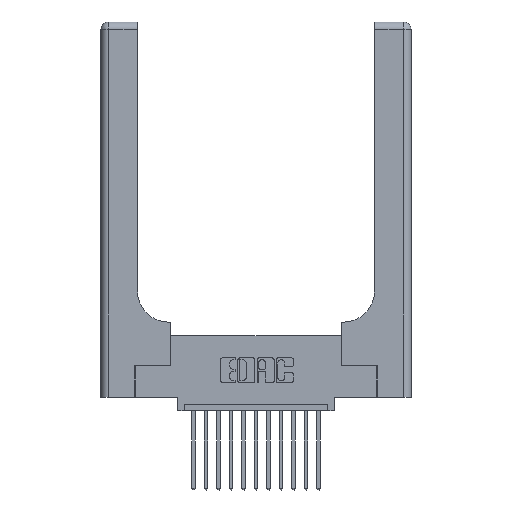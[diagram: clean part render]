
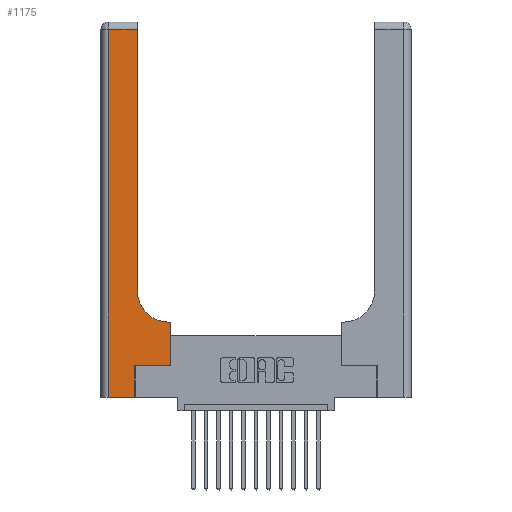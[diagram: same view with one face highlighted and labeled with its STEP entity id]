
A CAD part, top view. The second image highlights one B-rep face of the part: STEP entity #1175.
In plain terms, the highlighted planar face has unit normal (0, 0, 1).
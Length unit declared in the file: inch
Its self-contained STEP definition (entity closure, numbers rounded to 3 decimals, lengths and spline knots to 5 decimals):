
#129 = DIRECTION ( 'NONE',  ( 1., 0., 0. ) ) ;
#448 = PLANE ( 'NONE',  #14762 ) ;
#507 = DIRECTION ( 'NONE',  ( 0., 1., 0. ) ) ;
#669 = VECTOR ( 'NONE', #129, 39.37008 ) ;
#810 = VECTOR ( 'NONE', #507, 39.37008 ) ;
#836 = DIRECTION ( 'NONE',  ( 1., 0., 0. ) ) ;
#1175 = ADVANCED_FACE ( 'NONE', ( #10961 ), #448, .F. ) ;
#1431 = EDGE_CURVE ( 'NONE', #13646, #5494, #13086, .T. ) ;
#1509 = VECTOR ( 'NONE', #16615, 39.37008 ) ;
#1806 = ORIENTED_EDGE ( 'NONE', *, *, #9080, .T. ) ;
#1809 = DIRECTION ( 'NONE',  ( -1., 0., 0. ) ) ;
#2566 = DIRECTION ( 'NONE',  ( 1., 0., 0. ) ) ;
#2981 = VERTEX_POINT ( 'NONE', #3593 ) ;
#3011 = DIRECTION ( 'NONE',  ( 0., 0., -1. ) ) ;
#3562 = DIRECTION ( 'NONE',  ( 0., -1., 0. ) ) ;
#3593 = CARTESIAN_POINT ( 'NONE',  ( 0.06, 0., 0.37 ) ) ;
#3662 = VERTEX_POINT ( 'NONE', #6602 ) ;
#4334 = LINE ( 'NONE', #5508, #669 ) ;
#4370 = ORIENTED_EDGE ( 'NONE', *, *, #8007, .T. ) ;
#4672 = CARTESIAN_POINT ( 'NONE',  ( 0.2915, 3., 0.37 ) ) ;
#4741 = LINE ( 'NONE', #7735, #12445 ) ;
#5181 = EDGE_CURVE ( 'NONE', #10892, #3662, #14459, .T. ) ;
#5494 = VERTEX_POINT ( 'NONE', #14307 ) ;
#5508 = CARTESIAN_POINT ( 'NONE',  ( 0., 0., 0.37 ) ) ;
#5818 = CARTESIAN_POINT ( 'NONE',  ( 0.269, 0., 0.37 ) ) ;
#5832 = ORIENTED_EDGE ( 'NONE', *, *, #9420, .T. ) ;
#5854 = CARTESIAN_POINT ( 'NONE',  ( 0.5585, 0.6, 0.37 ) ) ;
#5992 = EDGE_CURVE ( 'NONE', #9072, #17401, #11463, .T. ) ;
#6553 = VECTOR ( 'NONE', #9749, 39.37008 ) ;
#6602 = CARTESIAN_POINT ( 'NONE',  ( 0.5415, 0.6, 0.37 ) ) ;
#7092 = VECTOR ( 'NONE', #9752, 39.37008 ) ;
#7735 = CARTESIAN_POINT ( 'NONE',  ( 0.06, 3., 0.37 ) ) ;
#7784 = LINE ( 'NONE', #11796, #16765 ) ;
#7988 = CARTESIAN_POINT ( 'NONE',  ( 0.5585, 0.25, 0.37 ) ) ;
#8007 = EDGE_CURVE ( 'NONE', #3662, #9575, #12531, .T. ) ;
#9072 = VERTEX_POINT ( 'NONE', #15487 ) ;
#9080 = EDGE_CURVE ( 'NONE', #15161, #10892, #15494, .T. ) ;
#9355 = ORIENTED_EDGE ( 'NONE', *, *, #5992, .T. ) ;
#9420 = EDGE_CURVE ( 'NONE', #17401, #15161, #7784, .T. ) ;
#9575 = VERTEX_POINT ( 'NONE', #13454 ) ;
#9749 = DIRECTION ( 'NONE',  ( -1., 0., 0. ) ) ;
#9752 = DIRECTION ( 'NONE',  ( -1., 0., 0. ) ) ;
#9813 = CARTESIAN_POINT ( 'NONE',  ( 0., 2.94, 0.37 ) ) ;
#9956 = ORIENTED_EDGE ( 'NONE', *, *, #15334, .T. ) ;
#10032 = CARTESIAN_POINT ( 'NONE',  ( 0., 3., 0.37 ) ) ;
#10176 = EDGE_CURVE ( 'NONE', #5494, #2981, #4741, .T. ) ;
#10892 = VERTEX_POINT ( 'NONE', #5854 ) ;
#10961 = FACE_OUTER_BOUND ( 'NONE', #15146, .T. ) ;
#11022 = VECTOR ( 'NONE', #16695, 39.37008 ) ;
#11345 = ORIENTED_EDGE ( 'NONE', *, *, #10176, .T. ) ;
#11414 = ORIENTED_EDGE ( 'NONE', *, *, #12075, .T. ) ;
#11463 = LINE ( 'NONE', #5818, #11022 ) ;
#11612 = CARTESIAN_POINT ( 'NONE',  ( 0.2915, 2.94, 0.37 ) ) ;
#11796 = CARTESIAN_POINT ( 'NONE',  ( 0.269, 0.25, 0.37 ) ) ;
#12075 = EDGE_CURVE ( 'NONE', #9575, #13646, #17129, .T. ) ;
#12445 = VECTOR ( 'NONE', #3562, 39.37008 ) ;
#12531 = CIRCLE ( 'NONE', #13778, 0.25 ) ;
#13086 = LINE ( 'NONE', #9813, #7092 ) ;
#13291 = ORIENTED_EDGE ( 'NONE', *, *, #5181, .T. ) ;
#13454 = CARTESIAN_POINT ( 'NONE',  ( 0.2915, 0.85, 0.37 ) ) ;
#13646 = VERTEX_POINT ( 'NONE', #11612 ) ;
#13778 = AXIS2_PLACEMENT_3D ( 'NONE', #14995, #17684, #2566 ) ;
#14307 = CARTESIAN_POINT ( 'NONE',  ( 0.06, 2.94, 0.37 ) ) ;
#14459 = LINE ( 'NONE', #14803, #6553 ) ;
#14762 = AXIS2_PLACEMENT_3D ( 'NONE', #10032, #3011, #1809 ) ;
#14803 = CARTESIAN_POINT ( 'NONE',  ( 0.2915, 0.6, 0.37 ) ) ;
#14995 = CARTESIAN_POINT ( 'NONE',  ( 0.5415, 0.85, 0.37 ) ) ;
#15146 = EDGE_LOOP ( 'NONE', ( #11414, #15822, #11345, #9956, #9355, #5832, #1806, #13291, #4370 ) ) ;
#15161 = VERTEX_POINT ( 'NONE', #7988 ) ;
#15334 = EDGE_CURVE ( 'NONE', #2981, #9072, #4334, .T. ) ;
#15487 = CARTESIAN_POINT ( 'NONE',  ( 0.269, 0., 0.37 ) ) ;
#15494 = LINE ( 'NONE', #16745, #1509 ) ;
#15822 = ORIENTED_EDGE ( 'NONE', *, *, #1431, .T. ) ;
#16120 = CARTESIAN_POINT ( 'NONE',  ( 0.269, 0.25, 0.37 ) ) ;
#16615 = DIRECTION ( 'NONE',  ( 0., 1., 0. ) ) ;
#16695 = DIRECTION ( 'NONE',  ( 0., 1., 0. ) ) ;
#16745 = CARTESIAN_POINT ( 'NONE',  ( 0.5585, 0.25, 0.37 ) ) ;
#16765 = VECTOR ( 'NONE', #836, 39.37008 ) ;
#17129 = LINE ( 'NONE', #4672, #810 ) ;
#17401 = VERTEX_POINT ( 'NONE', #16120 ) ;
#17684 = DIRECTION ( 'NONE',  ( 0., 0., -1. ) ) ;
